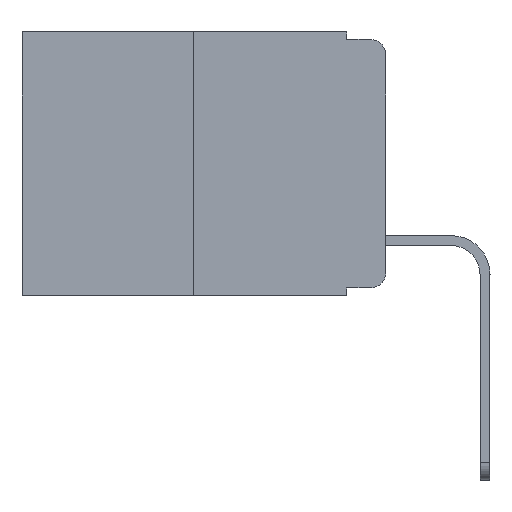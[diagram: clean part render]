
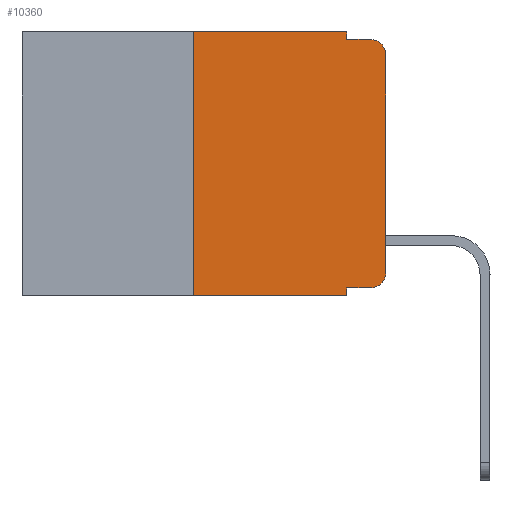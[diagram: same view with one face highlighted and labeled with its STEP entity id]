
A CAD part, left-side view. The second image highlights one B-rep face of the part: STEP entity #10360.
In plain terms, the highlighted planar face has unit normal (-1, 0, 0).
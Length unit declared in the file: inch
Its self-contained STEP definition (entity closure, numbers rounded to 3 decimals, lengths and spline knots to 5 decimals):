
#9 = LINE ( 'NONE', #1038, #11197 ) ;
#261 = CARTESIAN_POINT ( 'NONE',  ( 0., 0.051, -0.01 ) ) ;
#322 = CIRCLE ( 'NONE', #12263, 0.02 ) ;
#353 = ORIENTED_EDGE ( 'NONE', *, *, #3705, .F. ) ;
#359 = LINE ( 'NONE', #4784, #12010 ) ;
#571 = CARTESIAN_POINT ( 'NONE',  ( 0., 0.051, -0.343 ) ) ;
#826 = EDGE_CURVE ( 'NONE', #4272, #10180, #13010, .T. ) ;
#1038 = CARTESIAN_POINT ( 'NONE',  ( 0., 0.051, -0.01 ) ) ;
#1141 = EDGE_CURVE ( 'NONE', #10180, #12766, #3085, .T. ) ;
#1200 = LINE ( 'NONE', #10141, #10164 ) ;
#1364 = CARTESIAN_POINT ( 'NONE',  ( 0., 0., -0.03 ) ) ;
#1416 = ORIENTED_EDGE ( 'NONE', *, *, #11952, .F. ) ;
#1721 = CARTESIAN_POINT ( 'NONE',  ( 0., 0.02, -0.03 ) ) ;
#1947 = EDGE_CURVE ( 'NONE', #12766, #10919, #6358, .T. ) ;
#1975 = EDGE_CURVE ( 'NONE', #11690, #5793, #12810, .T. ) ;
#2264 = FACE_OUTER_BOUND ( 'NONE', #3315, .T. ) ;
#2594 = VECTOR ( 'NONE', #3550, 39.37008 ) ;
#2613 = VERTEX_POINT ( 'NONE', #8613 ) ;
#2703 = CARTESIAN_POINT ( 'NONE',  ( 0., 0.473, -0.343 ) ) ;
#3023 = VECTOR ( 'NONE', #5116, 39.37008 ) ;
#3085 = CIRCLE ( 'NONE', #5999, 0.02 ) ;
#3315 = EDGE_LOOP ( 'NONE', ( #5567, #12552, #8342, #353, #7379, #1416, #7050, #12899, #12039, #7453 ) ) ;
#3550 = DIRECTION ( 'NONE',  ( 0., 0., 1. ) ) ;
#3705 = EDGE_CURVE ( 'NONE', #12450, #10860, #7760, .T. ) ;
#4272 = VERTEX_POINT ( 'NONE', #8091 ) ;
#4471 = CARTESIAN_POINT ( 'NONE',  ( 0., 0., -0.313 ) ) ;
#4666 = DIRECTION ( 'NONE',  ( 0., 0., -1. ) ) ;
#4784 = CARTESIAN_POINT ( 'NONE',  ( 0., 0.051, 0. ) ) ;
#5025 = EDGE_CURVE ( 'NONE', #10860, #2613, #9, .T. ) ;
#5116 = DIRECTION ( 'NONE',  ( 0., 0., 1. ) ) ;
#5466 = CARTESIAN_POINT ( 'NONE',  ( 0., 0., 0. ) ) ;
#5567 = ORIENTED_EDGE ( 'NONE', *, *, #1947, .T. ) ;
#5793 = VERTEX_POINT ( 'NONE', #571 ) ;
#5999 = AXIS2_PLACEMENT_3D ( 'NONE', #7394, #9468, #4666 ) ;
#6358 = LINE ( 'NONE', #5466, #2594 ) ;
#6779 = CARTESIAN_POINT ( 'NONE',  ( 0., 0.25, -0.343 ) ) ;
#7017 = DIRECTION ( 'NONE',  ( 0., -1., 0. ) ) ;
#7050 = ORIENTED_EDGE ( 'NONE', *, *, #1975, .T. ) ;
#7245 = EDGE_CURVE ( 'NONE', #11117, #12450, #1200, .T. ) ;
#7379 = ORIENTED_EDGE ( 'NONE', *, *, #7245, .F. ) ;
#7394 = CARTESIAN_POINT ( 'NONE',  ( 0., 0.02, -0.313 ) ) ;
#7436 = DIRECTION ( 'NONE',  ( 0., 0., -1. ) ) ;
#7453 = ORIENTED_EDGE ( 'NONE', *, *, #1141, .T. ) ;
#7516 = CARTESIAN_POINT ( 'NONE',  ( 0., 0.473, 0. ) ) ;
#7760 = LINE ( 'NONE', #9379, #8549 ) ;
#8091 = CARTESIAN_POINT ( 'NONE',  ( 0., 0.051, -0.333 ) ) ;
#8256 = DIRECTION ( 'NONE',  ( 0., -1., 0. ) ) ;
#8342 = ORIENTED_EDGE ( 'NONE', *, *, #5025, .F. ) ;
#8549 = VECTOR ( 'NONE', #7436, 39.37008 ) ;
#8613 = CARTESIAN_POINT ( 'NONE',  ( 0., 0.02, -0.01 ) ) ;
#8776 = DIRECTION ( 'NONE',  ( 0., -1., 0. ) ) ;
#8927 = CARTESIAN_POINT ( 'NONE',  ( 0., 0.051, -0.333 ) ) ;
#9057 = AXIS2_PLACEMENT_3D ( 'NONE', #7516, #9598, #9640 ) ;
#9076 = VECTOR ( 'NONE', #9894, 39.37008 ) ;
#9222 = CARTESIAN_POINT ( 'NONE',  ( 0., 0.02, -0.333 ) ) ;
#9379 = CARTESIAN_POINT ( 'NONE',  ( 0., 0.051, 0. ) ) ;
#9468 = DIRECTION ( 'NONE',  ( -1., 0., 0. ) ) ;
#9598 = DIRECTION ( 'NONE',  ( 1., 0., 0. ) ) ;
#9640 = DIRECTION ( 'NONE',  ( 0., 0., -1. ) ) ;
#9715 = CARTESIAN_POINT ( 'NONE',  ( 0., 0.25, 0. ) ) ;
#9894 = DIRECTION ( 'NONE',  ( 0., -1., 0. ) ) ;
#10141 = CARTESIAN_POINT ( 'NONE',  ( 0., 0.473, 0. ) ) ;
#10164 = VECTOR ( 'NONE', #8256, 39.37008 ) ;
#10180 = VERTEX_POINT ( 'NONE', #9222 ) ;
#10360 = ADVANCED_FACE ( 'NONE', ( #2264 ), #11588, .F. ) ;
#10405 = LINE ( 'NONE', #11246, #3023 ) ;
#10860 = VERTEX_POINT ( 'NONE', #261 ) ;
#10919 = VERTEX_POINT ( 'NONE', #1364 ) ;
#10999 = DIRECTION ( 'NONE',  ( 0., 0., -1. ) ) ;
#11117 = VERTEX_POINT ( 'NONE', #9715 ) ;
#11166 = EDGE_CURVE ( 'NONE', #4272, #5793, #359, .T. ) ;
#11197 = VECTOR ( 'NONE', #7017, 39.37008 ) ;
#11246 = CARTESIAN_POINT ( 'NONE',  ( 0., 0.25, 0. ) ) ;
#11588 = PLANE ( 'NONE',  #9057 ) ;
#11690 = VERTEX_POINT ( 'NONE', #6779 ) ;
#11952 = EDGE_CURVE ( 'NONE', #11690, #11117, #10405, .T. ) ;
#12010 = VECTOR ( 'NONE', #10999, 39.37008 ) ;
#12039 = ORIENTED_EDGE ( 'NONE', *, *, #826, .T. ) ;
#12052 = CARTESIAN_POINT ( 'NONE',  ( 0., 0.051, 0. ) ) ;
#12263 = AXIS2_PLACEMENT_3D ( 'NONE', #1721, #12793, #12836 ) ;
#12273 = EDGE_CURVE ( 'NONE', #10919, #2613, #322, .T. ) ;
#12450 = VERTEX_POINT ( 'NONE', #12052 ) ;
#12552 = ORIENTED_EDGE ( 'NONE', *, *, #12273, .T. ) ;
#12766 = VERTEX_POINT ( 'NONE', #4471 ) ;
#12793 = DIRECTION ( 'NONE',  ( -1., 0., 0. ) ) ;
#12810 = LINE ( 'NONE', #2703, #12992 ) ;
#12836 = DIRECTION ( 'NONE',  ( 0., 0., -1. ) ) ;
#12899 = ORIENTED_EDGE ( 'NONE', *, *, #11166, .F. ) ;
#12992 = VECTOR ( 'NONE', #8776, 39.37008 ) ;
#13010 = LINE ( 'NONE', #8927, #9076 ) ;
